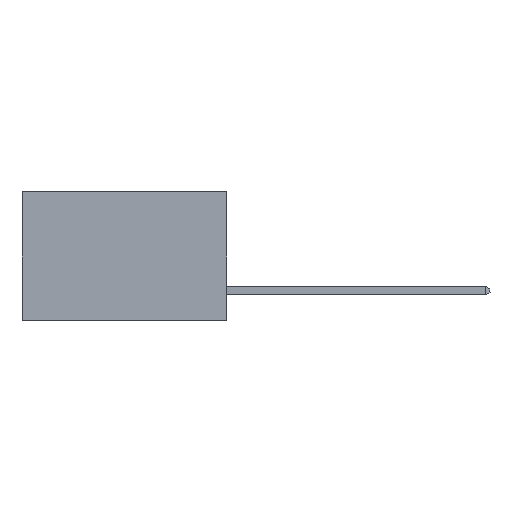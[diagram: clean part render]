
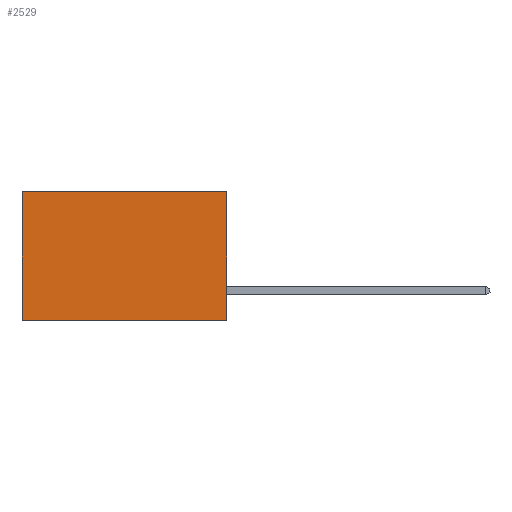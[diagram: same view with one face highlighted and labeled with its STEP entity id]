
A CAD part, left-side view. The second image highlights one B-rep face of the part: STEP entity #2529.
In plain terms, the highlighted planar face has unit normal (-1, 0, 0).
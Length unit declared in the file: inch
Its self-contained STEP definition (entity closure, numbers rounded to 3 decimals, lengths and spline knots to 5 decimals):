
#456 = DIRECTION ( 'NONE',  ( 0., 1., 0. ) ) ;
#599 = EDGE_CURVE ( 'NONE', #5331, #7763, #9645, .T. ) ;
#644 = DIRECTION ( 'NONE',  ( 0., 0., -1. ) ) ;
#817 = CARTESIAN_POINT ( 'NONE',  ( 0.277, 0., 0. ) ) ;
#1537 = VECTOR ( 'NONE', #644, 39.37008 ) ;
#2111 = VECTOR ( 'NONE', #456, 39.37008 ) ;
#2195 = CARTESIAN_POINT ( 'NONE',  ( 0.277, 0., -0.37 ) ) ;
#2529 = ADVANCED_FACE ( 'NONE', ( #4082 ), #9608, .F. ) ;
#3069 = CARTESIAN_POINT ( 'NONE',  ( 0.277, 0., -0.37 ) ) ;
#3244 = EDGE_CURVE ( 'NONE', #5877, #5331, #11219, .T. ) ;
#3281 = ORIENTED_EDGE ( 'NONE', *, *, #599, .T. ) ;
#4082 = FACE_OUTER_BOUND ( 'NONE', #10694, .T. ) ;
#4117 = EDGE_CURVE ( 'NONE', #8898, #7763, #7678, .T. ) ;
#4143 = EDGE_CURVE ( 'NONE', #5877, #8898, #12096, .T. ) ;
#4569 = CARTESIAN_POINT ( 'NONE',  ( 0.277, 0., -0.37 ) ) ;
#5113 = ORIENTED_EDGE ( 'NONE', *, *, #4117, .F. ) ;
#5331 = VERTEX_POINT ( 'NONE', #8920 ) ;
#5468 = ORIENTED_EDGE ( 'NONE', *, *, #4143, .F. ) ;
#5484 = ORIENTED_EDGE ( 'NONE', *, *, #3244, .T. ) ;
#5877 = VERTEX_POINT ( 'NONE', #11616 ) ;
#6251 = VECTOR ( 'NONE', #8747, 39.37008 ) ;
#6775 = CARTESIAN_POINT ( 'NONE',  ( 0.277, 0.59, -0.37 ) ) ;
#7678 = LINE ( 'NONE', #4569, #2111 ) ;
#7763 = VERTEX_POINT ( 'NONE', #6775 ) ;
#8747 = DIRECTION ( 'NONE',  ( 0., 1., 0. ) ) ;
#8773 = AXIS2_PLACEMENT_3D ( 'NONE', #3069, #10788, #10589 ) ;
#8898 = VERTEX_POINT ( 'NONE', #9606 ) ;
#8920 = CARTESIAN_POINT ( 'NONE',  ( 0.277, 0.59, 0. ) ) ;
#9606 = CARTESIAN_POINT ( 'NONE',  ( 0.277, 0., -0.37 ) ) ;
#9608 = PLANE ( 'NONE',  #8773 ) ;
#9645 = LINE ( 'NONE', #12311, #1537 ) ;
#10589 = DIRECTION ( 'NONE',  ( 0., 0., -1. ) ) ;
#10694 = EDGE_LOOP ( 'NONE', ( #3281, #5113, #5468, #5484 ) ) ;
#10788 = DIRECTION ( 'NONE',  ( 1., 0., 0. ) ) ;
#11219 = LINE ( 'NONE', #817, #6251 ) ;
#11616 = CARTESIAN_POINT ( 'NONE',  ( 0.277, 0., 0. ) ) ;
#11843 = VECTOR ( 'NONE', #12133, 39.37008 ) ;
#12096 = LINE ( 'NONE', #2195, #11843 ) ;
#12133 = DIRECTION ( 'NONE',  ( 0., 0., -1. ) ) ;
#12311 = CARTESIAN_POINT ( 'NONE',  ( 0.277, 0.59, -0.37 ) ) ;
